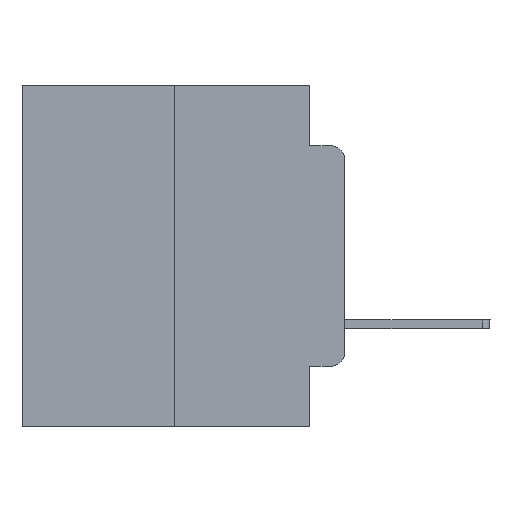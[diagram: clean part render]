
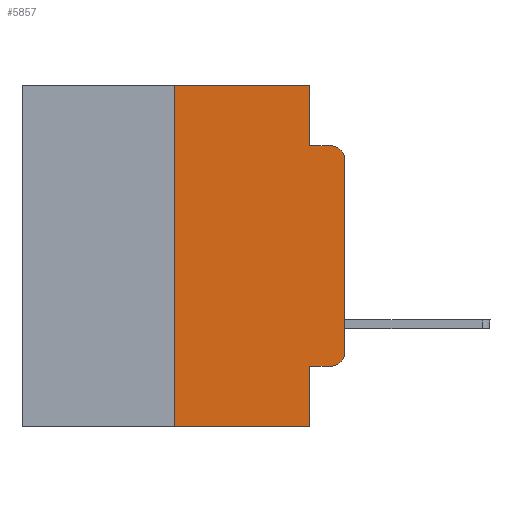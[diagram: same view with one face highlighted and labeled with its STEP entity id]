
A CAD part, left-side view. The second image highlights one B-rep face of the part: STEP entity #5857.
In plain terms, the highlighted planar face has unit normal (-1, 0, 0).
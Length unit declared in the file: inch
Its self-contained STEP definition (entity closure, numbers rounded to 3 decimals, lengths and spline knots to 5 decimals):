
#262 = VERTEX_POINT ( 'NONE', #15105 ) ;
#446 = EDGE_CURVE ( 'NONE', #6453, #9510, #10424, .T. ) ;
#468 = EDGE_CURVE ( 'NONE', #17538, #6371, #11966, .T. ) ;
#809 = VECTOR ( 'NONE', #19629, 39.37008 ) ;
#1150 = DIRECTION ( 'NONE',  ( 0., 0., 1. ) ) ;
#1419 = DIRECTION ( 'NONE',  ( 0., -1., 0. ) ) ;
#1727 = VERTEX_POINT ( 'NONE', #10557 ) ;
#2617 = CARTESIAN_POINT ( 'NONE',  ( 0., 0., -0.1085 ) ) ;
#2618 = CARTESIAN_POINT ( 'NONE',  ( 0., 0.02, -0.1085 ) ) ;
#2725 = DIRECTION ( 'NONE',  ( 0., 0., -1. ) ) ;
#3266 = CARTESIAN_POINT ( 'NONE',  ( 0., 0.051, -0.4115 ) ) ;
#3539 = CARTESIAN_POINT ( 'NONE',  ( 0., 0.051, -0.5 ) ) ;
#3749 = LINE ( 'NONE', #3266, #3860 ) ;
#3860 = VECTOR ( 'NONE', #1419, 39.37008 ) ;
#4049 = CARTESIAN_POINT ( 'NONE',  ( 0., 0., 0. ) ) ;
#4067 = DIRECTION ( 'NONE',  ( 0., -1., 0. ) ) ;
#4853 = CARTESIAN_POINT ( 'NONE',  ( 0., 0.25, -0.5 ) ) ;
#5069 = VERTEX_POINT ( 'NONE', #9972 ) ;
#5181 = VECTOR ( 'NONE', #18330, 39.37008 ) ;
#5249 = EDGE_CURVE ( 'NONE', #16598, #17538, #16720, .T. ) ;
#5325 = EDGE_CURVE ( 'NONE', #6453, #5069, #11511, .T. ) ;
#5587 = ORIENTED_EDGE ( 'NONE', *, *, #446, .T. ) ;
#5857 = ADVANCED_FACE ( 'NONE', ( #23187 ), #21251, .F. ) ;
#5954 = VECTOR ( 'NONE', #22412, 39.37008 ) ;
#6126 = CARTESIAN_POINT ( 'NONE',  ( 0., 0.051, 0. ) ) ;
#6371 = VERTEX_POINT ( 'NONE', #8740 ) ;
#6453 = VERTEX_POINT ( 'NONE', #4853 ) ;
#6460 = EDGE_LOOP ( 'NONE', ( #25332, #6498, #17354, #9135, #6625, #11158, #5587, #20118, #19701, #22027 ) ) ;
#6498 = ORIENTED_EDGE ( 'NONE', *, *, #25415, .T. ) ;
#6625 = ORIENTED_EDGE ( 'NONE', *, *, #15880, .F. ) ;
#7042 = EDGE_CURVE ( 'NONE', #1727, #19813, #3749, .T. ) ;
#7254 = DIRECTION ( 'NONE',  ( -1., 0., 0. ) ) ;
#7488 = DIRECTION ( 'NONE',  ( 0., 0., -1. ) ) ;
#8638 = EDGE_CURVE ( 'NONE', #19813, #262, #22387, .T. ) ;
#8740 = CARTESIAN_POINT ( 'NONE',  ( 0., 0.02, -0.0885 ) ) ;
#9135 = ORIENTED_EDGE ( 'NONE', *, *, #5249, .F. ) ;
#9510 = VERTEX_POINT ( 'NONE', #3539 ) ;
#9588 = VECTOR ( 'NONE', #1150, 39.37008 ) ;
#9972 = CARTESIAN_POINT ( 'NONE',  ( 0., 0.25, 0. ) ) ;
#10018 = CIRCLE ( 'NONE', #12525, 0.02 ) ;
#10340 = AXIS2_PLACEMENT_3D ( 'NONE', #13323, #7254, #11144 ) ;
#10407 = VECTOR ( 'NONE', #2725, 39.37008 ) ;
#10424 = LINE ( 'NONE', #12494, #16353 ) ;
#10557 = CARTESIAN_POINT ( 'NONE',  ( 0., 0.051, -0.4115 ) ) ;
#10894 = EDGE_CURVE ( 'NONE', #262, #15570, #13893, .T. ) ;
#11144 = DIRECTION ( 'NONE',  ( 0., 0., -1. ) ) ;
#11158 = ORIENTED_EDGE ( 'NONE', *, *, #5325, .F. ) ;
#11511 = LINE ( 'NONE', #17352, #9588 ) ;
#11966 = LINE ( 'NONE', #20438, #5181 ) ;
#12494 = CARTESIAN_POINT ( 'NONE',  ( 0., 0.473, -0.5 ) ) ;
#12519 = CARTESIAN_POINT ( 'NONE',  ( 0., 0.473, 0. ) ) ;
#12525 = AXIS2_PLACEMENT_3D ( 'NONE', #2618, #22475, #20401 ) ;
#13174 = DIRECTION ( 'NONE',  ( 1., 0., 0. ) ) ;
#13323 = CARTESIAN_POINT ( 'NONE',  ( 0., 0.02, -0.3915 ) ) ;
#13893 = LINE ( 'NONE', #4049, #809 ) ;
#15105 = CARTESIAN_POINT ( 'NONE',  ( 0., 0., -0.3915 ) ) ;
#15570 = VERTEX_POINT ( 'NONE', #2617 ) ;
#15772 = CARTESIAN_POINT ( 'NONE',  ( 0., 0.051, -0.0885 ) ) ;
#15880 = EDGE_CURVE ( 'NONE', #5069, #16598, #20463, .T. ) ;
#16353 = VECTOR ( 'NONE', #4067, 39.37008 ) ;
#16492 = LINE ( 'NONE', #6126, #23582 ) ;
#16598 = VERTEX_POINT ( 'NONE', #21819 ) ;
#16720 = LINE ( 'NONE', #18532, #10407 ) ;
#17352 = CARTESIAN_POINT ( 'NONE',  ( 0., 0.25, 0. ) ) ;
#17354 = ORIENTED_EDGE ( 'NONE', *, *, #468, .F. ) ;
#17538 = VERTEX_POINT ( 'NONE', #15772 ) ;
#18330 = DIRECTION ( 'NONE',  ( 0., -1., 0. ) ) ;
#18532 = CARTESIAN_POINT ( 'NONE',  ( 0., 0.051, 0. ) ) ;
#18835 = CARTESIAN_POINT ( 'NONE',  ( 0., 0.02, -0.4115 ) ) ;
#19629 = DIRECTION ( 'NONE',  ( 0., 0., 1. ) ) ;
#19701 = ORIENTED_EDGE ( 'NONE', *, *, #7042, .T. ) ;
#19813 = VERTEX_POINT ( 'NONE', #18835 ) ;
#20118 = ORIENTED_EDGE ( 'NONE', *, *, #22433, .F. ) ;
#20401 = DIRECTION ( 'NONE',  ( 0., 0., -1. ) ) ;
#20438 = CARTESIAN_POINT ( 'NONE',  ( 0., 0.051, -0.0885 ) ) ;
#20463 = LINE ( 'NONE', #12519, #5954 ) ;
#21251 = PLANE ( 'NONE',  #24555 ) ;
#21819 = CARTESIAN_POINT ( 'NONE',  ( 0., 0.051, 0. ) ) ;
#22027 = ORIENTED_EDGE ( 'NONE', *, *, #8638, .T. ) ;
#22387 = CIRCLE ( 'NONE', #10340, 0.02 ) ;
#22412 = DIRECTION ( 'NONE',  ( 0., -1., 0. ) ) ;
#22433 = EDGE_CURVE ( 'NONE', #1727, #9510, #16492, .T. ) ;
#22475 = DIRECTION ( 'NONE',  ( -1., 0., 0. ) ) ;
#23187 = FACE_OUTER_BOUND ( 'NONE', #6460, .T. ) ;
#23582 = VECTOR ( 'NONE', #24442, 39.37008 ) ;
#24442 = DIRECTION ( 'NONE',  ( 0., 0., -1. ) ) ;
#24555 = AXIS2_PLACEMENT_3D ( 'NONE', #25021, #13174, #7488 ) ;
#25021 = CARTESIAN_POINT ( 'NONE',  ( 0., 0.473, 0. ) ) ;
#25332 = ORIENTED_EDGE ( 'NONE', *, *, #10894, .T. ) ;
#25415 = EDGE_CURVE ( 'NONE', #15570, #6371, #10018, .T. ) ;
